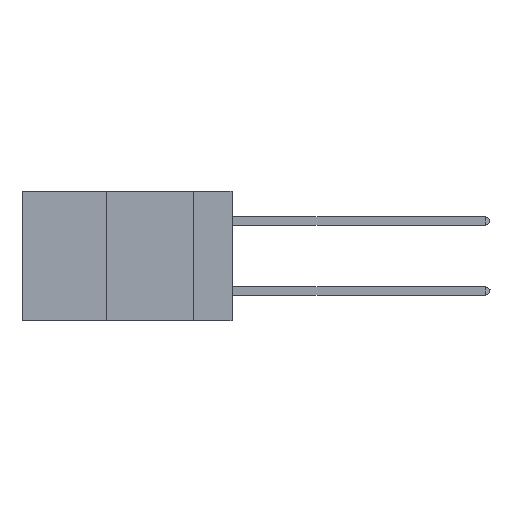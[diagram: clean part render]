
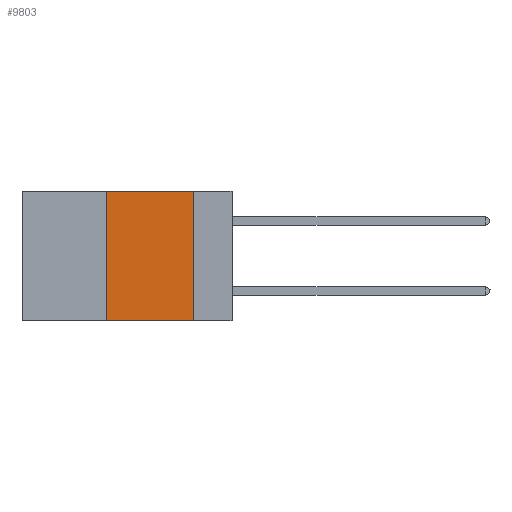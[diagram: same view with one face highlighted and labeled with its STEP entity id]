
A CAD part, left-side view. The second image highlights one B-rep face of the part: STEP entity #9803.
In plain terms, the highlighted planar face has unit normal (-1, 0, 0).
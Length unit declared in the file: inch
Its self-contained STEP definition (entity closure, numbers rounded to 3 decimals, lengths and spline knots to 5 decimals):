
#1467 = CARTESIAN_POINT ( 'NONE',  ( 0., 0.11, -0.37 ) ) ;
#1611 = CARTESIAN_POINT ( 'NONE',  ( 0., 0.11, 0. ) ) ;
#1712 = VERTEX_POINT ( 'NONE', #1467 ) ;
#3478 = VECTOR ( 'NONE', #12217, 39.37008 ) ;
#4384 = EDGE_CURVE ( 'NONE', #35436, #1712, #12771, .T. ) ;
#5167 = CARTESIAN_POINT ( 'NONE',  ( 0., 0.6, 0. ) ) ;
#5474 = VECTOR ( 'NONE', #19721, 39.37008 ) ;
#6149 = EDGE_CURVE ( 'NONE', #34862, #35436, #20568, .T. ) ;
#7395 = AXIS2_PLACEMENT_3D ( 'NONE', #5167, #34337, #16708 ) ;
#7467 = EDGE_CURVE ( 'NONE', #26276, #34862, #20572, .T. ) ;
#8003 = PLANE ( 'NONE',  #7395 ) ;
#8168 = CARTESIAN_POINT ( 'NONE',  ( 0., 0.6, -0.37 ) ) ;
#9002 = CARTESIAN_POINT ( 'NONE',  ( 0., 0.6, 0. ) ) ;
#9803 = ADVANCED_FACE ( 'NONE', ( #10847 ), #8003, .F. ) ;
#10847 = FACE_OUTER_BOUND ( 'NONE', #34746, .T. ) ;
#12217 = DIRECTION ( 'NONE',  ( 0., 0., -1. ) ) ;
#12332 = ORIENTED_EDGE ( 'NONE', *, *, #6149, .F. ) ;
#12485 = CARTESIAN_POINT ( 'NONE',  ( 0., 0.36, -0.37 ) ) ;
#12771 = LINE ( 'NONE', #36107, #3478 ) ;
#13343 = VECTOR ( 'NONE', #35363, 39.37008 ) ;
#14699 = CARTESIAN_POINT ( 'NONE',  ( 0., 0.36, 0. ) ) ;
#16708 = DIRECTION ( 'NONE',  ( 0., 0., -1. ) ) ;
#19721 = DIRECTION ( 'NONE',  ( 0., -1., 0. ) ) ;
#20568 = LINE ( 'NONE', #9002, #34476 ) ;
#20572 = LINE ( 'NONE', #14699, #13343 ) ;
#26276 = VERTEX_POINT ( 'NONE', #12485 ) ;
#27074 = ORIENTED_EDGE ( 'NONE', *, *, #27328, .T. ) ;
#27328 = EDGE_CURVE ( 'NONE', #26276, #1712, #34136, .T. ) ;
#32417 = CARTESIAN_POINT ( 'NONE',  ( 0., 0.36, 0. ) ) ;
#34136 = LINE ( 'NONE', #8168, #5474 ) ;
#34337 = DIRECTION ( 'NONE',  ( 1., 0., 0. ) ) ;
#34476 = VECTOR ( 'NONE', #35359, 39.37008 ) ;
#34518 = ORIENTED_EDGE ( 'NONE', *, *, #7467, .F. ) ;
#34746 = EDGE_LOOP ( 'NONE', ( #35551, #12332, #34518, #27074 ) ) ;
#34862 = VERTEX_POINT ( 'NONE', #32417 ) ;
#35359 = DIRECTION ( 'NONE',  ( 0., -1., 0. ) ) ;
#35363 = DIRECTION ( 'NONE',  ( 0., 0., 1. ) ) ;
#35436 = VERTEX_POINT ( 'NONE', #1611 ) ;
#35551 = ORIENTED_EDGE ( 'NONE', *, *, #4384, .F. ) ;
#36107 = CARTESIAN_POINT ( 'NONE',  ( 0., 0.11, 0. ) ) ;
